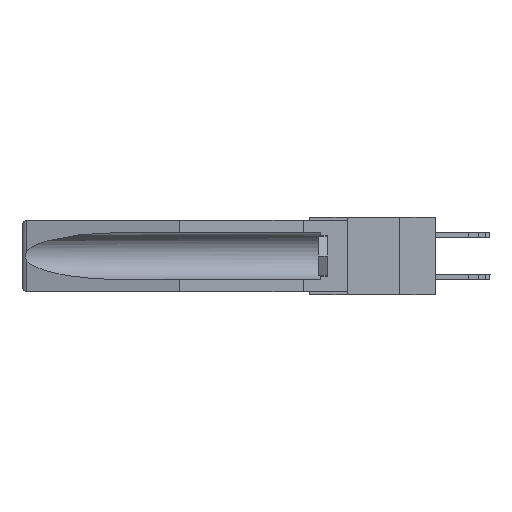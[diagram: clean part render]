
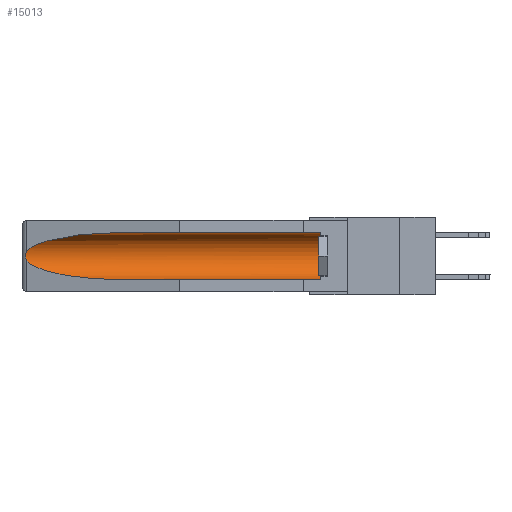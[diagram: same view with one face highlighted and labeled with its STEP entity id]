
A CAD part, left-side view. The second image highlights one B-rep face of the part: STEP entity #15013.
In plain terms, the highlighted cylindrical face has radius 2.857 mm (diameter 5.715 mm), a partial arc.
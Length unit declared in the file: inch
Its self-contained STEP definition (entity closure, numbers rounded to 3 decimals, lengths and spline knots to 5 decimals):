
#152 = CARTESIAN_POINT ( 'NONE',  ( 0.26597, 1.52961, -0.15275 ) ) ;
#219 = CARTESIAN_POINT ( 'NONE',  ( 0.2673, 1.5327, -0.16383 ) ) ;
#289 = ORIENTED_EDGE ( 'NONE', *, *, #7850, .T. ) ;
#1060 = CARTESIAN_POINT ( 'NONE',  ( 0.155, -0.30754, -0.059 ) ) ;
#1445 = CARTESIAN_POINT ( 'NONE',  ( 0.21114, 1.30732, -0.059 ) ) ;
#2096 = LINE ( 'NONE', #1060, #6508 ) ;
#2195 = CARTESIAN_POINT ( 'NONE',  ( 0.2673, 1.53269, -0.17917 ) ) ;
#2553 = CARTESIAN_POINT ( 'NONE',  ( 0.26537, 1.52718, -0.19328 ) ) ;
#2930 = ORIENTED_EDGE ( 'NONE', *, *, #9053, .T. ) ;
#3572 = CARTESIAN_POINT ( 'NONE',  ( 0.155, -0.30754, -0.1715 ) ) ;
#4273 = VERTEX_POINT ( 'NONE', #17987 ) ;
#4730 = EDGE_CURVE ( 'NONE', #10535, #17426, #12817, .T. ) ;
#4940 = CARTESIAN_POINT ( 'NONE',  ( 0.2675, 1.53308, -0.16763 ) ) ;
#5376 = EDGE_CURVE ( 'NONE', #8732, #10535, #18546, .T. ) ;
#5453 = ORIENTED_EDGE ( 'NONE', *, *, #5376, .T. ) ;
#5901 = DIRECTION ( 'NONE',  ( 0., 1., 0. ) ) ;
#6508 = VECTOR ( 'NONE', #5901, 39.37008 ) ;
#6575 = DIRECTION ( 'NONE',  ( 0., 1., 0. ) ) ;
#6961 = CARTESIAN_POINT ( 'NONE',  ( 0.155, -0.30754, -0.284 ) ) ;
#7309 = CYLINDRICAL_SURFACE ( 'NONE', #12687, 0.1125 ) ;
#7542 = CARTESIAN_POINT ( 'NONE',  ( 0.25451, 1.48313, -0.09465 ) ) ;
#7579 = DIRECTION ( 'NONE',  ( 0., 0., 1. ) ) ;
#7713 = VECTOR ( 'NONE', #12039, 39.37008 ) ;
#7850 = EDGE_CURVE ( 'NONE', #4273, #15271, #9476, .T. ) ;
#7899 = ORIENTED_EDGE ( 'NONE', *, *, #8420, .F. ) ;
#8012 = CARTESIAN_POINT ( 'NONE',  ( 0.26654, 1.53092, -0.15636 ) ) ;
#8292 = CARTESIAN_POINT ( 'NONE',  ( 0.2675, 1.53308, -0.17534 ) ) ;
#8420 = EDGE_CURVE ( 'NONE', #4273, #12733, #14861, .T. ) ;
#8467 = CARTESIAN_POINT ( 'NONE',  ( 0.26537, 1.52718, -0.14972 ) ) ;
#8732 = VERTEX_POINT ( 'NONE', #15795 ) ;
#9053 = EDGE_CURVE ( 'NONE', #17426, #12733, #11288, .T. ) ;
#9476 = CIRCLE ( 'NONE', #19642, 0.1125 ) ;
#10210 = CARTESIAN_POINT ( 'NONE',  ( 0.25451, 1.48313, -0.24835 ) ) ;
#10253 = FACE_OUTER_BOUND ( 'NONE', #14511, .T. ) ;
#10368 = ORIENTED_EDGE ( 'NONE', *, *, #4730, .T. ) ;
#10535 = VERTEX_POINT ( 'NONE', #8467 ) ;
#11288 =( BOUNDED_CURVE ( )  B_SPLINE_CURVE ( 3, ( #2553, #10210, #15085, #11928 ),
 .UNSPECIFIED., .F., .F. ) 
 B_SPLINE_CURVE_WITH_KNOTS ( ( 4, 4 ),
 ( 0.1948, 1.5708 ),
 .UNSPECIFIED. ) 
 CURVE ( )  GEOMETRIC_REPRESENTATION_ITEM ( )  RATIONAL_B_SPLINE_CURVE ( ( 1., 0.848, 0.848, 1. ) ) 
 REPRESENTATION_ITEM ( '' )  );
#11928 = CARTESIAN_POINT ( 'NONE',  ( 0.155, 1.07973, -0.284 ) ) ;
#12039 = DIRECTION ( 'NONE',  ( 0., 1., 0. ) ) ;
#12258 = ORIENTED_EDGE ( 'NONE', *, *, #17293, .T. ) ;
#12537 = CARTESIAN_POINT ( 'NONE',  ( 0.26537, 1.52718, -0.19328 ) ) ;
#12687 = AXIS2_PLACEMENT_3D ( 'NONE', #3572, #6575, #17515 ) ;
#12733 = VERTEX_POINT ( 'NONE', #13774 ) ;
#12817 = B_SPLINE_CURVE_WITH_KNOTS ( 'NONE', 3,
 ( #17332, #152, #8012, #219, #4940, #8292, #2195, #19223, #17856, #16309 ),
 .UNSPECIFIED., .F., .F.,
 ( 4, 2, 2, 2, 4 ),
 ( 0., 0.00029, 0.00058, 0.00087, 0.00117 ),
 .UNSPECIFIED. ) ;
#13774 = CARTESIAN_POINT ( 'NONE',  ( 0.155, 1.07973, -0.284 ) ) ;
#14029 = DIRECTION ( 'NONE',  ( 0., -1., 0. ) ) ;
#14511 = EDGE_LOOP ( 'NONE', ( #5453, #10368, #2930, #7899, #289, #12258 ) ) ;
#14861 = LINE ( 'NONE', #6961, #7713 ) ;
#14995 = CARTESIAN_POINT ( 'NONE',  ( 0.155, 0.126, -0.059 ) ) ;
#15013 = ADVANCED_FACE ( 'NONE', ( #10253 ), #7309, .F. ) ;
#15085 = CARTESIAN_POINT ( 'NONE',  ( 0.21114, 1.30732, -0.284 ) ) ;
#15271 = VERTEX_POINT ( 'NONE', #14995 ) ;
#15795 = CARTESIAN_POINT ( 'NONE',  ( 0.155, 1.07973, -0.059 ) ) ;
#16309 = CARTESIAN_POINT ( 'NONE',  ( 0.26537, 1.52718, -0.19328 ) ) ;
#17070 = CARTESIAN_POINT ( 'NONE',  ( 0.26537, 1.52718, -0.14972 ) ) ;
#17134 = CARTESIAN_POINT ( 'NONE',  ( 0.155, 1.07973, -0.059 ) ) ;
#17293 = EDGE_CURVE ( 'NONE', #15271, #8732, #2096, .T. ) ;
#17332 = CARTESIAN_POINT ( 'NONE',  ( 0.26537, 1.52718, -0.14972 ) ) ;
#17426 = VERTEX_POINT ( 'NONE', #12537 ) ;
#17515 = DIRECTION ( 'NONE',  ( 0., 0., 1. ) ) ;
#17856 = CARTESIAN_POINT ( 'NONE',  ( 0.26597, 1.5296, -0.19026 ) ) ;
#17987 = CARTESIAN_POINT ( 'NONE',  ( 0.155, 0.126, -0.284 ) ) ;
#18546 =( BOUNDED_CURVE ( )  B_SPLINE_CURVE ( 3, ( #17134, #1445, #7542, #17070 ),
 .UNSPECIFIED., .F., .F. ) 
 B_SPLINE_CURVE_WITH_KNOTS ( ( 4, 4 ),
 ( 4.71239, 6.08839 ),
 .UNSPECIFIED. ) 
 CURVE ( )  GEOMETRIC_REPRESENTATION_ITEM ( )  RATIONAL_B_SPLINE_CURVE ( ( 1., 0.848, 0.848, 1. ) ) 
 REPRESENTATION_ITEM ( '' )  );
#19223 = CARTESIAN_POINT ( 'NONE',  ( 0.26655, 1.53094, -0.18657 ) ) ;
#19642 = AXIS2_PLACEMENT_3D ( 'NONE', #20140, #14029, #7579 ) ;
#20140 = CARTESIAN_POINT ( 'NONE',  ( 0.155, 0.126, -0.1715 ) ) ;
